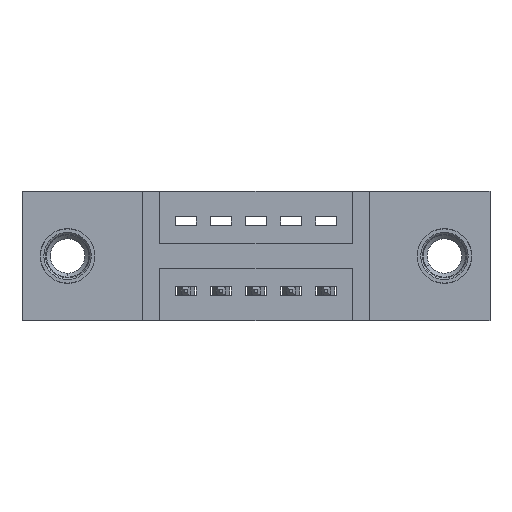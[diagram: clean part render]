
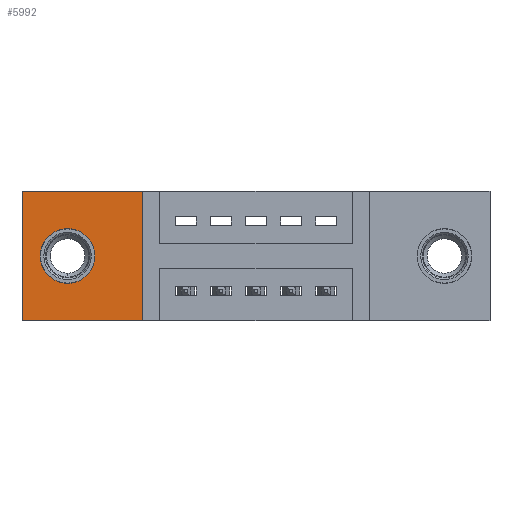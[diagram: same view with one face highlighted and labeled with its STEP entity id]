
A CAD part, front view. The second image highlights one B-rep face of the part: STEP entity #5992.
In plain terms, the highlighted planar face has unit normal (0, -1, 0).
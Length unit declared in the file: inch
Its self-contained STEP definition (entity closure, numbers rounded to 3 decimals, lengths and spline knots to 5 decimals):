
#210 = VECTOR ( 'NONE', #9422, 39.37008 ) ;
#225 = EDGE_CURVE ( 'NONE', #711, #6593, #7895, .T. ) ;
#234 = DIRECTION ( 'NONE',  ( 0., 0., -1. ) ) ;
#554 = ORIENTED_EDGE ( 'NONE', *, *, #1383, .T. ) ;
#711 = VERTEX_POINT ( 'NONE', #7182 ) ;
#798 = ORIENTED_EDGE ( 'NONE', *, *, #3495, .F. ) ;
#831 = CIRCLE ( 'NONE', #7569, 0.078 ) ;
#929 = DIRECTION ( 'NONE',  ( 1., 0., 0. ) ) ;
#930 = ORIENTED_EDGE ( 'NONE', *, *, #2635, .T. ) ;
#1123 = CARTESIAN_POINT ( 'NONE',  ( 0., 0.17, -0.37 ) ) ;
#1339 = CARTESIAN_POINT ( 'NONE',  ( 0., 0.17, -0.37 ) ) ;
#1371 = DIRECTION ( 'NONE',  ( 0., -1., 0. ) ) ;
#1383 = EDGE_CURVE ( 'NONE', #1610, #5472, #5664, .T. ) ;
#1610 = VERTEX_POINT ( 'NONE', #1339 ) ;
#1627 = DIRECTION ( 'NONE',  ( 0., -1., 0. ) ) ;
#1783 = CARTESIAN_POINT ( 'NONE',  ( 0., 0.17, 0. ) ) ;
#2332 = FACE_OUTER_BOUND ( 'NONE', #9602, .T. ) ;
#2340 = VECTOR ( 'NONE', #2633, 39.37008 ) ;
#2354 = VECTOR ( 'NONE', #929, 39.37008 ) ;
#2633 = DIRECTION ( 'NONE',  ( -1., 0., 0. ) ) ;
#2635 = EDGE_CURVE ( 'NONE', #2970, #9795, #6716, .T. ) ;
#2970 = VERTEX_POINT ( 'NONE', #7629 ) ;
#3234 = CARTESIAN_POINT ( 'NONE',  ( 0.13, 0.17, -0.185 ) ) ;
#3423 = CARTESIAN_POINT ( 'NONE',  ( 0., 0.17, 0. ) ) ;
#3495 = EDGE_CURVE ( 'NONE', #6593, #711, #831, .T. ) ;
#4025 = ORIENTED_EDGE ( 'NONE', *, *, #9558, .T. ) ;
#4511 = DIRECTION ( 'NONE',  ( 0., -1., 0. ) ) ;
#4677 = FACE_BOUND ( 'NONE', #8474, .T. ) ;
#4800 = AXIS2_PLACEMENT_3D ( 'NONE', #3234, #1627, #234 ) ;
#5472 = VERTEX_POINT ( 'NONE', #7662 ) ;
#5664 = LINE ( 'NONE', #1123, #2354 ) ;
#5992 = ADVANCED_FACE ( 'NONE', ( #4677, #2332 ), #6785, .T. ) ;
#6176 = CARTESIAN_POINT ( 'NONE',  ( 0.13, 0.17, -0.185 ) ) ;
#6537 = ORIENTED_EDGE ( 'NONE', *, *, #7650, .T. ) ;
#6593 = VERTEX_POINT ( 'NONE', #8895 ) ;
#6716 = LINE ( 'NONE', #1783, #2340 ) ;
#6777 = CARTESIAN_POINT ( 'NONE',  ( 0., 0.17, 0. ) ) ;
#6785 = PLANE ( 'NONE',  #7085 ) ;
#6811 = VECTOR ( 'NONE', #8338, 39.37008 ) ;
#6929 = DIRECTION ( 'NONE',  ( 0., 0., -1. ) ) ;
#7057 = LINE ( 'NONE', #7619, #6811 ) ;
#7085 = AXIS2_PLACEMENT_3D ( 'NONE', #8975, #4511, #9701 ) ;
#7182 = CARTESIAN_POINT ( 'NONE',  ( 0.13, 0.17, -0.263 ) ) ;
#7569 = AXIS2_PLACEMENT_3D ( 'NONE', #6176, #1371, #6929 ) ;
#7619 = CARTESIAN_POINT ( 'NONE',  ( 0.3425, 0.17, 0. ) ) ;
#7629 = CARTESIAN_POINT ( 'NONE',  ( 0.3425, 0.17, 0. ) ) ;
#7650 = EDGE_CURVE ( 'NONE', #5472, #2970, #7057, .T. ) ;
#7662 = CARTESIAN_POINT ( 'NONE',  ( 0.3425, 0.17, -0.37 ) ) ;
#7851 = ORIENTED_EDGE ( 'NONE', *, *, #225, .F. ) ;
#7895 = CIRCLE ( 'NONE', #4800, 0.078 ) ;
#8338 = DIRECTION ( 'NONE',  ( 0., 0., 1. ) ) ;
#8474 = EDGE_LOOP ( 'NONE', ( #798, #7851 ) ) ;
#8579 = LINE ( 'NONE', #3423, #210 ) ;
#8895 = CARTESIAN_POINT ( 'NONE',  ( 0.13, 0.17, -0.107 ) ) ;
#8975 = CARTESIAN_POINT ( 'NONE',  ( 0., 0.17, -0.37 ) ) ;
#9422 = DIRECTION ( 'NONE',  ( 0., 0., -1. ) ) ;
#9558 = EDGE_CURVE ( 'NONE', #9795, #1610, #8579, .T. ) ;
#9602 = EDGE_LOOP ( 'NONE', ( #4025, #554, #6537, #930 ) ) ;
#9701 = DIRECTION ( 'NONE',  ( 0., 0., -1. ) ) ;
#9795 = VERTEX_POINT ( 'NONE', #6777 ) ;
